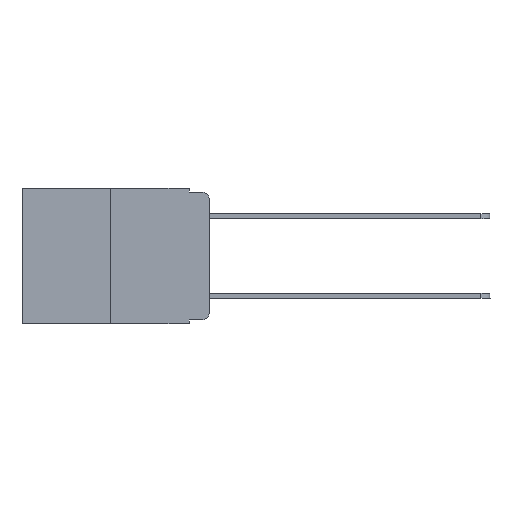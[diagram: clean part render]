
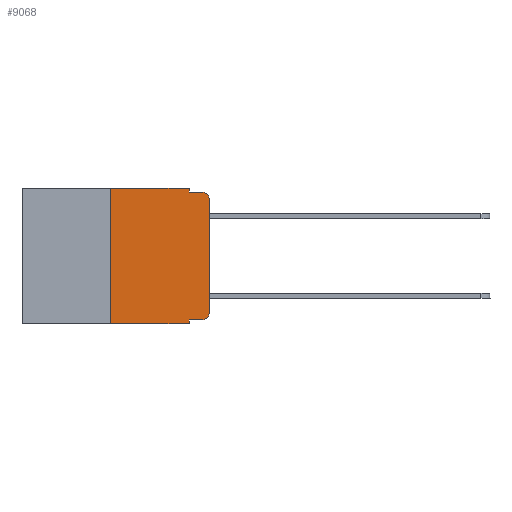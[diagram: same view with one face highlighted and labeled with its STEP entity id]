
A CAD part, left-side view. The second image highlights one B-rep face of the part: STEP entity #9068.
In plain terms, the highlighted planar face has unit normal (-1, 0, 0).
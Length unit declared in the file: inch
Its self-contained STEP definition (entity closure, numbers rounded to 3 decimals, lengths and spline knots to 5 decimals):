
#70 = DIRECTION ( 'NONE',  ( 0., -1., 0. ) ) ;
#383 = CARTESIAN_POINT ( 'NONE',  ( 0., 0.473, 0. ) ) ;
#412 = DIRECTION ( 'NONE',  ( 0., -1., 0. ) ) ;
#437 = EDGE_CURVE ( 'NONE', #2548, #8496, #1619, .T. ) ;
#687 = ORIENTED_EDGE ( 'NONE', *, *, #7856, .F. ) ;
#693 = CARTESIAN_POINT ( 'NONE',  ( 0., 0., 0. ) ) ;
#772 = VECTOR ( 'NONE', #70, 39.37008 ) ;
#792 = CIRCLE ( 'NONE', #6525, 0.02 ) ;
#957 = LINE ( 'NONE', #4100, #3083 ) ;
#970 = CARTESIAN_POINT ( 'NONE',  ( 0., 0.051, -0.01 ) ) ;
#1080 = CARTESIAN_POINT ( 'NONE',  ( 0., 0.02, -0.333 ) ) ;
#1186 = LINE ( 'NONE', #1385, #3900 ) ;
#1217 = CARTESIAN_POINT ( 'NONE',  ( 0., 0., -0.03 ) ) ;
#1337 = DIRECTION ( 'NONE',  ( 0., -1., 0. ) ) ;
#1343 = CARTESIAN_POINT ( 'NONE',  ( 0., 0.02, -0.313 ) ) ;
#1385 = CARTESIAN_POINT ( 'NONE',  ( 0., 0.473, 0. ) ) ;
#1619 = CIRCLE ( 'NONE', #1782, 0.02 ) ;
#1704 = EDGE_CURVE ( 'NONE', #9481, #9387, #8600, .T. ) ;
#1782 = AXIS2_PLACEMENT_3D ( 'NONE', #7259, #6274, #2513 ) ;
#2211 = LINE ( 'NONE', #3128, #6735 ) ;
#2441 = ORIENTED_EDGE ( 'NONE', *, *, #6373, .T. ) ;
#2513 = DIRECTION ( 'NONE',  ( 0., 0., -1. ) ) ;
#2548 = VERTEX_POINT ( 'NONE', #1217 ) ;
#3083 = VECTOR ( 'NONE', #3320, 39.37008 ) ;
#3128 = CARTESIAN_POINT ( 'NONE',  ( 0., 0.051, -0.01 ) ) ;
#3180 = CARTESIAN_POINT ( 'NONE',  ( 0., 0.051, 0. ) ) ;
#3320 = DIRECTION ( 'NONE',  ( 0., -1., 0. ) ) ;
#3450 = CARTESIAN_POINT ( 'NONE',  ( 0., 0.25, 0. ) ) ;
#3475 = CARTESIAN_POINT ( 'NONE',  ( 0., 0.051, 0. ) ) ;
#3900 = VECTOR ( 'NONE', #412, 39.37008 ) ;
#4028 = VECTOR ( 'NONE', #5494, 39.37008 ) ;
#4100 = CARTESIAN_POINT ( 'NONE',  ( 0., 0.473, -0.343 ) ) ;
#4354 = ORIENTED_EDGE ( 'NONE', *, *, #437, .T. ) ;
#4467 = CARTESIAN_POINT ( 'NONE',  ( 0., 0., -0.313 ) ) ;
#4584 = EDGE_CURVE ( 'NONE', #9481, #7270, #7939, .T. ) ;
#4634 = ORIENTED_EDGE ( 'NONE', *, *, #4584, .T. ) ;
#4739 = VERTEX_POINT ( 'NONE', #4467 ) ;
#5125 = ORIENTED_EDGE ( 'NONE', *, *, #7412, .T. ) ;
#5233 = VECTOR ( 'NONE', #7755, 39.37008 ) ;
#5372 = VERTEX_POINT ( 'NONE', #7025 ) ;
#5494 = DIRECTION ( 'NONE',  ( 0., 0., -1. ) ) ;
#5595 = EDGE_CURVE ( 'NONE', #5372, #7682, #1186, .T. ) ;
#5752 = CARTESIAN_POINT ( 'NONE',  ( 0., 0.02, -0.01 ) ) ;
#5919 = VERTEX_POINT ( 'NONE', #970 ) ;
#5953 = DIRECTION ( 'NONE',  ( 0., 0., 1. ) ) ;
#6230 = AXIS2_PLACEMENT_3D ( 'NONE', #383, #9034, #9943 ) ;
#6274 = DIRECTION ( 'NONE',  ( -1., 0., 0. ) ) ;
#6373 = EDGE_CURVE ( 'NONE', #6702, #9387, #957, .T. ) ;
#6525 = AXIS2_PLACEMENT_3D ( 'NONE', #1343, #6786, #7574 ) ;
#6702 = VERTEX_POINT ( 'NONE', #9590 ) ;
#6735 = VECTOR ( 'NONE', #1337, 39.37008 ) ;
#6786 = DIRECTION ( 'NONE',  ( -1., 0., 0. ) ) ;
#6803 = PLANE ( 'NONE',  #6230 ) ;
#6956 = EDGE_CURVE ( 'NONE', #4739, #2548, #7787, .T. ) ;
#7025 = CARTESIAN_POINT ( 'NONE',  ( 0., 0.25, 0. ) ) ;
#7259 = CARTESIAN_POINT ( 'NONE',  ( 0., 0.02, -0.03 ) ) ;
#7270 = VERTEX_POINT ( 'NONE', #1080 ) ;
#7412 = EDGE_CURVE ( 'NONE', #7270, #4739, #792, .T. ) ;
#7574 = DIRECTION ( 'NONE',  ( 0., 0., -1. ) ) ;
#7682 = VERTEX_POINT ( 'NONE', #3475 ) ;
#7755 = DIRECTION ( 'NONE',  ( 0., 0., -1. ) ) ;
#7787 = LINE ( 'NONE', #693, #10174 ) ;
#7856 = EDGE_CURVE ( 'NONE', #7682, #5919, #8578, .T. ) ;
#7891 = CARTESIAN_POINT ( 'NONE',  ( 0., 0.051, -0.333 ) ) ;
#7939 = LINE ( 'NONE', #7891, #772 ) ;
#8083 = ORIENTED_EDGE ( 'NONE', *, *, #5595, .F. ) ;
#8131 = LINE ( 'NONE', #3450, #9508 ) ;
#8160 = EDGE_LOOP ( 'NONE', ( #8207, #4354, #8949, #687, #8083, #8405, #2441, #9796, #4634, #5125 ) ) ;
#8207 = ORIENTED_EDGE ( 'NONE', *, *, #6956, .T. ) ;
#8256 = FACE_OUTER_BOUND ( 'NONE', #8160, .T. ) ;
#8342 = CARTESIAN_POINT ( 'NONE',  ( 0., 0.051, -0.333 ) ) ;
#8405 = ORIENTED_EDGE ( 'NONE', *, *, #8502, .F. ) ;
#8407 = DIRECTION ( 'NONE',  ( 0., 0., 1. ) ) ;
#8496 = VERTEX_POINT ( 'NONE', #5752 ) ;
#8502 = EDGE_CURVE ( 'NONE', #6702, #5372, #8131, .T. ) ;
#8578 = LINE ( 'NONE', #9440, #5233 ) ;
#8600 = LINE ( 'NONE', #3180, #4028 ) ;
#8949 = ORIENTED_EDGE ( 'NONE', *, *, #9946, .F. ) ;
#9034 = DIRECTION ( 'NONE',  ( 1., 0., 0. ) ) ;
#9068 = ADVANCED_FACE ( 'NONE', ( #8256 ), #6803, .F. ) ;
#9387 = VERTEX_POINT ( 'NONE', #9535 ) ;
#9440 = CARTESIAN_POINT ( 'NONE',  ( 0., 0.051, 0. ) ) ;
#9481 = VERTEX_POINT ( 'NONE', #8342 ) ;
#9508 = VECTOR ( 'NONE', #5953, 39.37008 ) ;
#9535 = CARTESIAN_POINT ( 'NONE',  ( 0., 0.051, -0.343 ) ) ;
#9590 = CARTESIAN_POINT ( 'NONE',  ( 0., 0.25, -0.343 ) ) ;
#9796 = ORIENTED_EDGE ( 'NONE', *, *, #1704, .F. ) ;
#9943 = DIRECTION ( 'NONE',  ( 0., 0., -1. ) ) ;
#9946 = EDGE_CURVE ( 'NONE', #5919, #8496, #2211, .T. ) ;
#10174 = VECTOR ( 'NONE', #8407, 39.37008 ) ;
